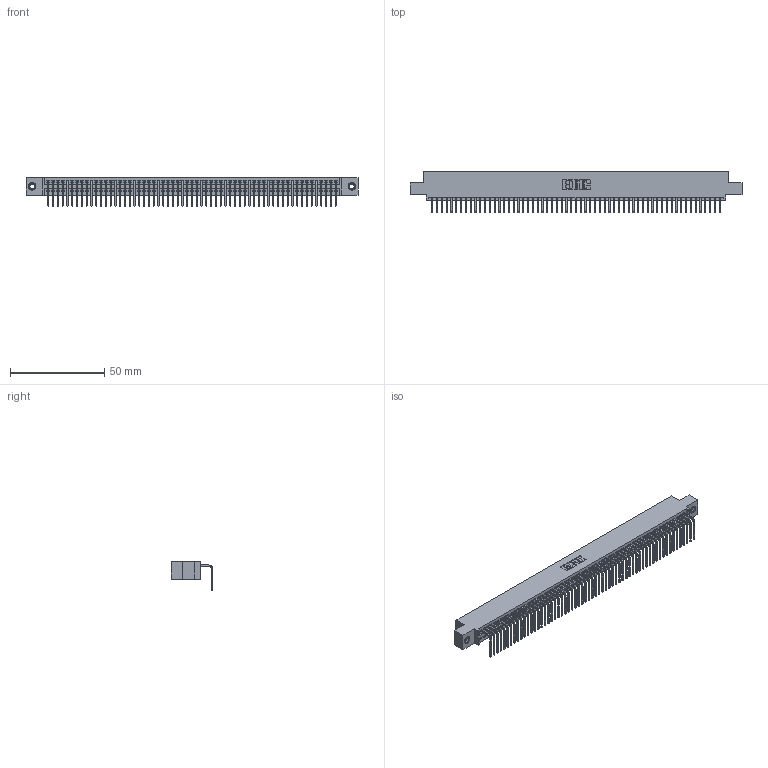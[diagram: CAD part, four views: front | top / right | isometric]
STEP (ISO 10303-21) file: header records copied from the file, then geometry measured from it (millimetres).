
FILE_DESCRIPTION (( 'STEP AP203' ), '1' );
FILE_NAME ('395-061-558-407.STEP', '2018-11-23T23:10:22', ( '' ), ( '' ), 'SwSTEP 2.0', 'SolidWorks 2016', '' );
FILE_SCHEMA (( 'CONFIG_CONTROL_DESIGN' ));
Length unit declared in the file: inch
Products named in the file (4): 345 Part_0.110 Offset - 0.156 Dia-TI; 395-061-558-407; 345-292-001_558 Tail - 2; 345-250-001_345-250-005-103
Assembly tree (64 placements, depth 2):
  395-061-558-407
    345 Part_0.110 Offset - 0.156 Dia-TI
    345-292-001_558 Tail - 2  x61
    345-250-001_345-250-005-103  x2
Bounding box: 176.15 x 21.83 x 15.37 mm (x, y, z)
Volume: 17002.8 mm3; surface area: 24162.1 mm2
Topology: 64 solids, 64 shells, 3850 faces, 11591 edges, 7638 vertices
Faces by surface type: plane 2678, cylinder 1156, cone 12, torus 4
Entity records: 44754 total; most frequent: CARTESIAN_POINT 7734, ORIENTED_EDGE 7722, DIRECTION 6753, EDGE_CURVE 3861, VECTOR 3465, LINE 3465, VERTEX_POINT 2568, AXIS2_PLACEMENT_3D 1644
